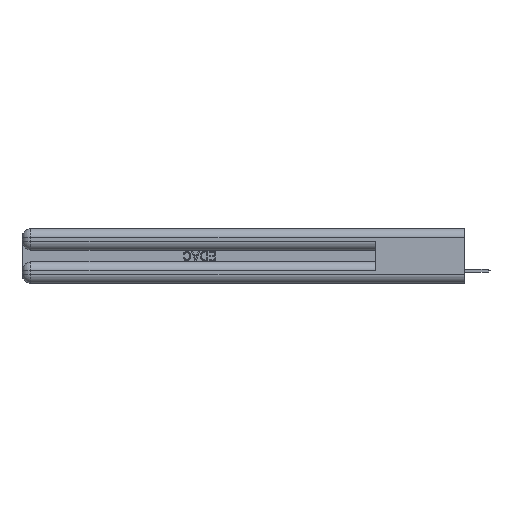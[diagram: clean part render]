
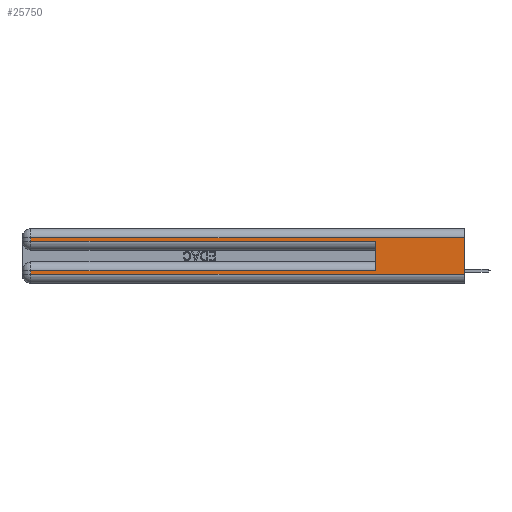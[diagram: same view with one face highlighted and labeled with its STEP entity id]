
A CAD part, left-side view. The second image highlights one B-rep face of the part: STEP entity #25750.
In plain terms, the highlighted planar face has unit normal (-1, 0, 0).
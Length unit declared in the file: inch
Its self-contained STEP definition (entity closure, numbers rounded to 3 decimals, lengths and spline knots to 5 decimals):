
#452 = DIRECTION ( 'NONE',  ( 0., 0., 1. ) ) ;
#572 = VERTEX_POINT ( 'NONE', #16556 ) ;
#873 = VECTOR ( 'NONE', #15032, 39.37008 ) ;
#2133 = EDGE_CURVE ( 'NONE', #25729, #4477, #12049, .T. ) ;
#2875 = VERTEX_POINT ( 'NONE', #12830 ) ;
#3141 = LINE ( 'NONE', #31714, #28429 ) ;
#3507 = CARTESIAN_POINT ( 'NONE',  ( 0., 0., 0.06 ) ) ;
#3977 = DIRECTION ( 'NONE',  ( 0., -1., 0. ) ) ;
#4477 = VERTEX_POINT ( 'NONE', #37385 ) ;
#5000 = EDGE_CURVE ( 'NONE', #2875, #25729, #34059, .T. ) ;
#6560 = AXIS2_PLACEMENT_3D ( 'NONE', #33137, #36402, #33287 ) ;
#7942 = CARTESIAN_POINT ( 'NONE',  ( 0., 2.94, 0.37 ) ) ;
#7996 = CARTESIAN_POINT ( 'NONE',  ( 0., 0., 0.31 ) ) ;
#8086 = ORIENTED_EDGE ( 'NONE', *, *, #2133, .T. ) ;
#8264 = CARTESIAN_POINT ( 'NONE',  ( 0., 0., 0.085 ) ) ;
#10347 = CARTESIAN_POINT ( 'NONE',  ( 0., 0.6, 0.145 ) ) ;
#10720 = VECTOR ( 'NONE', #452, 39.37008 ) ;
#11221 = DIRECTION ( 'NONE',  ( 0., 1., 0. ) ) ;
#12049 = LINE ( 'NONE', #7942, #15615 ) ;
#12140 = ORIENTED_EDGE ( 'NONE', *, *, #5000, .T. ) ;
#12830 = CARTESIAN_POINT ( 'NONE',  ( 0., 0., 0.31 ) ) ;
#14587 = LINE ( 'NONE', #34310, #873 ) ;
#15032 = DIRECTION ( 'NONE',  ( 0., -1., 0. ) ) ;
#15122 = VECTOR ( 'NONE', #3977, 39.37008 ) ;
#15615 = VECTOR ( 'NONE', #30956, 39.37008 ) ;
#15999 = ORIENTED_EDGE ( 'NONE', *, *, #26010, .T. ) ;
#16556 = CARTESIAN_POINT ( 'NONE',  ( 0., 2.94, 0.085 ) ) ;
#16922 = ORIENTED_EDGE ( 'NONE', *, *, #26304, .F. ) ;
#20169 = ORIENTED_EDGE ( 'NONE', *, *, #36692, .F. ) ;
#22880 = EDGE_CURVE ( 'NONE', #41363, #41162, #33698, .T. ) ;
#23761 = VECTOR ( 'NONE', #40765, 39.37008 ) ;
#23879 = LINE ( 'NONE', #8264, #35986 ) ;
#24131 = PLANE ( 'NONE',  #6560 ) ;
#25729 = VERTEX_POINT ( 'NONE', #39089 ) ;
#25750 = ADVANCED_FACE ( 'NONE', ( #29466 ), #24131, .F. ) ;
#26010 = EDGE_CURVE ( 'NONE', #40605, #572, #23879, .T. ) ;
#26304 = EDGE_CURVE ( 'NONE', #40605, #39039, #29916, .T. ) ;
#27519 = ORIENTED_EDGE ( 'NONE', *, *, #35514, .T. ) ;
#28429 = VECTOR ( 'NONE', #34413, 39.37008 ) ;
#29466 = FACE_OUTER_BOUND ( 'NONE', #31033, .T. ) ;
#29916 = LINE ( 'NONE', #10347, #10720 ) ;
#30153 = CARTESIAN_POINT ( 'NONE',  ( 0., 0.6, 0.085 ) ) ;
#30956 = DIRECTION ( 'NONE',  ( 0., 0., -1. ) ) ;
#31033 = EDGE_LOOP ( 'NONE', ( #20169, #12140, #8086, #31845, #16922, #15999, #27519, #38850 ) ) ;
#31714 = CARTESIAN_POINT ( 'NONE',  ( 0., 0., 0.37 ) ) ;
#31756 = EDGE_CURVE ( 'NONE', #4477, #39039, #14587, .T. ) ;
#31845 = ORIENTED_EDGE ( 'NONE', *, *, #31756, .T. ) ;
#32512 = VECTOR ( 'NONE', #36343, 39.37008 ) ;
#33137 = CARTESIAN_POINT ( 'NONE',  ( 0., 0., 0.37 ) ) ;
#33287 = DIRECTION ( 'NONE',  ( 0., 0., -1. ) ) ;
#33353 = LINE ( 'NONE', #39829, #23761 ) ;
#33590 = CARTESIAN_POINT ( 'NONE',  ( 0., 2.94, 0.06 ) ) ;
#33698 = LINE ( 'NONE', #39410, #15122 ) ;
#34059 = LINE ( 'NONE', #7996, #32512 ) ;
#34310 = CARTESIAN_POINT ( 'NONE',  ( 0., 0., 0.285 ) ) ;
#34413 = DIRECTION ( 'NONE',  ( 0., 0., -1. ) ) ;
#34687 = CARTESIAN_POINT ( 'NONE',  ( 0., 0.6, 0.285 ) ) ;
#35514 = EDGE_CURVE ( 'NONE', #572, #41363, #33353, .T. ) ;
#35986 = VECTOR ( 'NONE', #11221, 39.37008 ) ;
#36343 = DIRECTION ( 'NONE',  ( 0., 1., 0. ) ) ;
#36402 = DIRECTION ( 'NONE',  ( 1., 0., 0. ) ) ;
#36692 = EDGE_CURVE ( 'NONE', #2875, #41162, #3141, .T. ) ;
#37385 = CARTESIAN_POINT ( 'NONE',  ( 0., 2.94, 0.285 ) ) ;
#38850 = ORIENTED_EDGE ( 'NONE', *, *, #22880, .T. ) ;
#39039 = VERTEX_POINT ( 'NONE', #34687 ) ;
#39089 = CARTESIAN_POINT ( 'NONE',  ( 0., 2.94, 0.31 ) ) ;
#39410 = CARTESIAN_POINT ( 'NONE',  ( 0., 0., 0.06 ) ) ;
#39829 = CARTESIAN_POINT ( 'NONE',  ( 0., 2.94, 0.37 ) ) ;
#40605 = VERTEX_POINT ( 'NONE', #30153 ) ;
#40765 = DIRECTION ( 'NONE',  ( 0., 0., -1. ) ) ;
#41162 = VERTEX_POINT ( 'NONE', #3507 ) ;
#41363 = VERTEX_POINT ( 'NONE', #33590 ) ;
